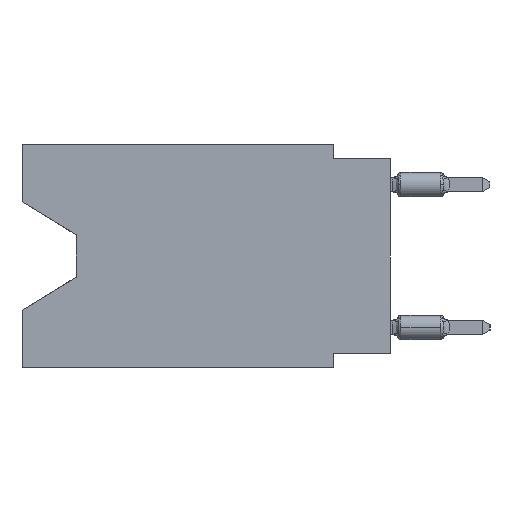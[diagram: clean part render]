
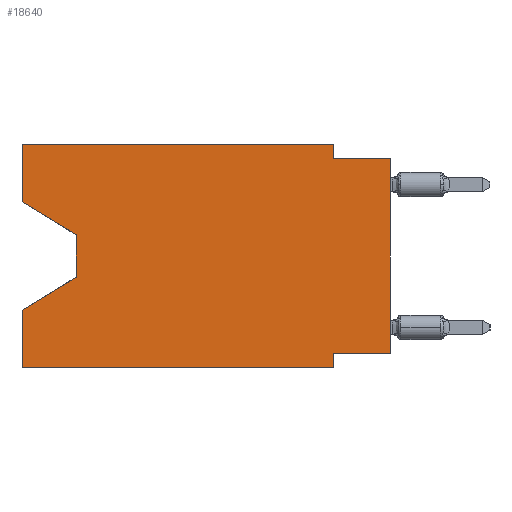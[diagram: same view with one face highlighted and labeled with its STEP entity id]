
A CAD part, left-side view. The second image highlights one B-rep face of the part: STEP entity #18640.
In plain terms, the highlighted planar face has unit normal (-1, 0, 0).
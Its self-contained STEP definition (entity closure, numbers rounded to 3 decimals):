
#350 = CARTESIAN_POINT ( 'NONE',  ( 0., 0., -0.635 ) ) ;
#1340 = EDGE_CURVE ( 'NONE', #52031, #31484, #19507, .T. ) ;
#1582 = DIRECTION ( 'NONE',  ( 0., -1., 0. ) ) ;
#2026 = VERTEX_POINT ( 'NONE', #47717 ) ;
#2382 = VECTOR ( 'NONE', #40360, 1000. ) ;
#2469 = VERTEX_POINT ( 'NONE', #350 ) ;
#3065 = ORIENTED_EDGE ( 'NONE', *, *, #46610, .T. ) ;
#3108 = LINE ( 'NONE', #36503, #32228 ) ;
#4371 = LINE ( 'NONE', #38327, #32671 ) ;
#5145 = VECTOR ( 'NONE', #49472, 1000. ) ;
#6347 = LINE ( 'NONE', #19965, #5145 ) ;
#6784 = CARTESIAN_POINT ( 'NONE',  ( 0., 0., -9.271 ) ) ;
#7745 = DIRECTION ( 'NONE',  ( 0., 0., -1. ) ) ;
#7906 = ORIENTED_EDGE ( 'NONE', *, *, #29679, .T. ) ;
#8065 = DIRECTION ( 'NONE',  ( 0., 0.855, -0.519 ) ) ;
#8136 = ORIENTED_EDGE ( 'NONE', *, *, #33522, .F. ) ;
#8181 = VERTEX_POINT ( 'NONE', #45275 ) ;
#8781 = CARTESIAN_POINT ( 'NONE',  ( 0., 2.54, 0. ) ) ;
#10425 = CARTESIAN_POINT ( 'NONE',  ( 0., 2.54, -0.635 ) ) ;
#10652 = LINE ( 'NONE', #39596, #13589 ) ;
#11776 = VERTEX_POINT ( 'NONE', #27442 ) ;
#13589 = VECTOR ( 'NONE', #14266, 1000. ) ;
#14266 = DIRECTION ( 'NONE',  ( 0., 0., -1. ) ) ;
#15043 = ORIENTED_EDGE ( 'NONE', *, *, #31019, .T. ) ;
#16184 = DIRECTION ( 'NONE',  ( 0., 0., 1. ) ) ;
#16324 = ORIENTED_EDGE ( 'NONE', *, *, #53104, .T. ) ;
#18640 = ADVANCED_FACE ( 'NONE', ( #43263 ), #43821, .F. ) ;
#18702 = EDGE_CURVE ( 'NONE', #8181, #51681, #44089, .T. ) ;
#18976 = VERTEX_POINT ( 'NONE', #26425 ) ;
#19507 = LINE ( 'NONE', #53475, #47782 ) ;
#19965 = CARTESIAN_POINT ( 'NONE',  ( 0., 13.97, -4.013 ) ) ;
#20511 = VERTEX_POINT ( 'NONE', #47074 ) ;
#21073 = DIRECTION ( 'NONE',  ( 0., -0.855, -0.519 ) ) ;
#21720 = VECTOR ( 'NONE', #8065, 1000. ) ;
#22211 = CARTESIAN_POINT ( 'NONE',  ( 0., 2.54, -9.271 ) ) ;
#22238 = ORIENTED_EDGE ( 'NONE', *, *, #26978, .T. ) ;
#23080 = EDGE_CURVE ( 'NONE', #2026, #52031, #53555, .T. ) ;
#23446 = ORIENTED_EDGE ( 'NONE', *, *, #46238, .F. ) ;
#23880 = EDGE_CURVE ( 'NONE', #31484, #48178, #37532, .T. ) ;
#24802 = AXIS2_PLACEMENT_3D ( 'NONE', #30741, #52164, #39631 ) ;
#26425 = CARTESIAN_POINT ( 'NONE',  ( 0., 13.97, -4.013 ) ) ;
#26978 = EDGE_CURVE ( 'NONE', #54127, #20511, #33399, .T. ) ;
#27442 = CARTESIAN_POINT ( 'NONE',  ( 0., 2.54, -9.906 ) ) ;
#27608 = CARTESIAN_POINT ( 'NONE',  ( 0., 16.383, -9.906 ) ) ;
#29679 = EDGE_CURVE ( 'NONE', #18976, #54127, #6347, .T. ) ;
#30422 = VECTOR ( 'NONE', #7745, 1000. ) ;
#30741 = CARTESIAN_POINT ( 'NONE',  ( 0., 16.383, 0. ) ) ;
#30918 = ORIENTED_EDGE ( 'NONE', *, *, #23880, .F. ) ;
#31019 = EDGE_CURVE ( 'NONE', #2026, #18976, #4371, .T. ) ;
#31484 = VERTEX_POINT ( 'NONE', #50253 ) ;
#32228 = VECTOR ( 'NONE', #53211, 1000. ) ;
#32671 = VECTOR ( 'NONE', #21073, 1000. ) ;
#33399 = LINE ( 'NONE', #33670, #21720 ) ;
#33522 = EDGE_CURVE ( 'NONE', #43501, #20511, #44050, .T. ) ;
#33573 = ORIENTED_EDGE ( 'NONE', *, *, #1340, .F. ) ;
#33670 = CARTESIAN_POINT ( 'NONE',  ( 0., 13.97, -5.893 ) ) ;
#35276 = EDGE_LOOP ( 'NONE', ( #15043, #7906, #22238, #8136, #3065, #53025, #39948, #16324, #23446, #30918, #33573, #40988 ) ) ;
#35634 = LINE ( 'NONE', #52618, #2382 ) ;
#36358 = CARTESIAN_POINT ( 'NONE',  ( 0., 0., -0.635 ) ) ;
#36503 = CARTESIAN_POINT ( 'NONE',  ( 0., 16.383, -9.906 ) ) ;
#36563 = DIRECTION ( 'NONE',  ( 0., 1., 0. ) ) ;
#37532 = LINE ( 'NONE', #8781, #30422 ) ;
#38149 = VECTOR ( 'NONE', #16184, 1000. ) ;
#38327 = CARTESIAN_POINT ( 'NONE',  ( 0., 16.383, -2.546 ) ) ;
#39055 = EDGE_CURVE ( 'NONE', #51681, #11776, #10652, .T. ) ;
#39571 = DIRECTION ( 'NONE',  ( 0., -1., 0. ) ) ;
#39596 = CARTESIAN_POINT ( 'NONE',  ( 0., 2.54, -9.906 ) ) ;
#39631 = DIRECTION ( 'NONE',  ( 0., 0., -1. ) ) ;
#39860 = CARTESIAN_POINT ( 'NONE',  ( 0., 16.383, 0. ) ) ;
#39948 = ORIENTED_EDGE ( 'NONE', *, *, #18702, .F. ) ;
#39981 = LINE ( 'NONE', #36358, #41237 ) ;
#40360 = DIRECTION ( 'NONE',  ( 0., 0., 1. ) ) ;
#40988 = ORIENTED_EDGE ( 'NONE', *, *, #23080, .F. ) ;
#41119 = CARTESIAN_POINT ( 'NONE',  ( 0., 16.383, 0. ) ) ;
#41237 = VECTOR ( 'NONE', #1582, 1000. ) ;
#41852 = DIRECTION ( 'NONE',  ( 0., 0., 1. ) ) ;
#43263 = FACE_OUTER_BOUND ( 'NONE', #35276, .T. ) ;
#43501 = VERTEX_POINT ( 'NONE', #27608 ) ;
#43821 = PLANE ( 'NONE',  #24802 ) ;
#44050 = LINE ( 'NONE', #39860, #38149 ) ;
#44089 = LINE ( 'NONE', #6784, #44359 ) ;
#44359 = VECTOR ( 'NONE', #36563, 1000. ) ;
#45275 = CARTESIAN_POINT ( 'NONE',  ( 0., 0., -9.271 ) ) ;
#46238 = EDGE_CURVE ( 'NONE', #48178, #2469, #39981, .T. ) ;
#46610 = EDGE_CURVE ( 'NONE', #43501, #11776, #3108, .T. ) ;
#47074 = CARTESIAN_POINT ( 'NONE',  ( 0., 16.383, -7.36 ) ) ;
#47717 = CARTESIAN_POINT ( 'NONE',  ( 0., 16.383, -2.546 ) ) ;
#47782 = VECTOR ( 'NONE', #39571, 1000. ) ;
#48178 = VERTEX_POINT ( 'NONE', #10425 ) ;
#49129 = VECTOR ( 'NONE', #41852, 1000. ) ;
#49472 = DIRECTION ( 'NONE',  ( 0., 0., -1. ) ) ;
#50200 = CARTESIAN_POINT ( 'NONE',  ( 0., 16.383, 0. ) ) ;
#50253 = CARTESIAN_POINT ( 'NONE',  ( 0., 2.54, 0. ) ) ;
#51681 = VERTEX_POINT ( 'NONE', #22211 ) ;
#51810 = CARTESIAN_POINT ( 'NONE',  ( 0., 13.97, -5.893 ) ) ;
#52031 = VERTEX_POINT ( 'NONE', #41119 ) ;
#52164 = DIRECTION ( 'NONE',  ( 1., 0., 0. ) ) ;
#52618 = CARTESIAN_POINT ( 'NONE',  ( 0., 0., 0. ) ) ;
#53025 = ORIENTED_EDGE ( 'NONE', *, *, #39055, .F. ) ;
#53104 = EDGE_CURVE ( 'NONE', #8181, #2469, #35634, .T. ) ;
#53211 = DIRECTION ( 'NONE',  ( 0., -1., 0. ) ) ;
#53475 = CARTESIAN_POINT ( 'NONE',  ( 0., 16.383, 0. ) ) ;
#53555 = LINE ( 'NONE', #50200, #49129 ) ;
#54127 = VERTEX_POINT ( 'NONE', #51810 ) ;
